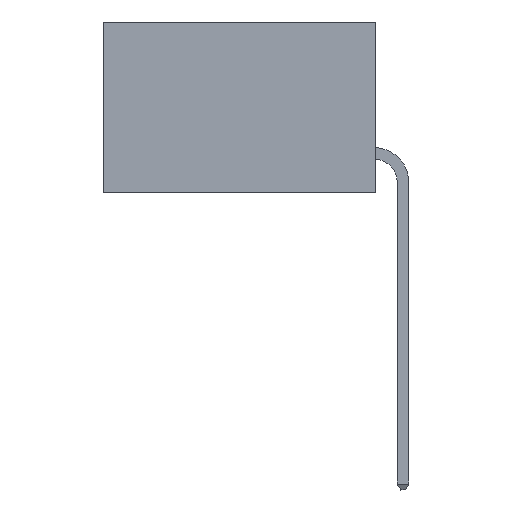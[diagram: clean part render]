
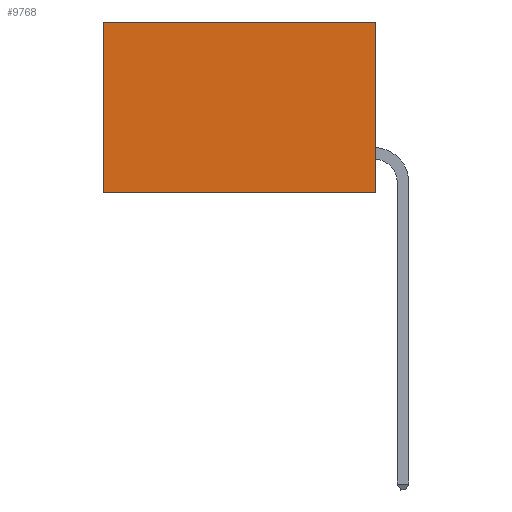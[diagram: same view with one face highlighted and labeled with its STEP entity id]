
A CAD part, left-side view. The second image highlights one B-rep face of the part: STEP entity #9768.
In plain terms, the highlighted planar face has unit normal (-1, 0, 0).
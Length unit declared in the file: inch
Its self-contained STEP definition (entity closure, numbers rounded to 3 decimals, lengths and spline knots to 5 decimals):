
#250 = EDGE_LOOP ( 'NONE', ( #1846, #6431, #14286, #9051 ) ) ;
#856 = VERTEX_POINT ( 'NONE', #9621 ) ;
#1846 = ORIENTED_EDGE ( 'NONE', *, *, #5291, .T. ) ;
#2152 = CARTESIAN_POINT ( 'NONE',  ( 0.277, 0., -0.37 ) ) ;
#2549 = CARTESIAN_POINT ( 'NONE',  ( 0.277, 0., -0.37 ) ) ;
#2844 = CARTESIAN_POINT ( 'NONE',  ( 0.277, 0., -0.37 ) ) ;
#3000 = CARTESIAN_POINT ( 'NONE',  ( 0.277, 0., -0.37 ) ) ;
#3125 = LINE ( 'NONE', #2844, #11781 ) ;
#3521 = VERTEX_POINT ( 'NONE', #2152 ) ;
#3768 = CARTESIAN_POINT ( 'NONE',  ( 0.277, 0.59, -0.37 ) ) ;
#4004 = DIRECTION ( 'NONE',  ( 0., 0., -1. ) ) ;
#4199 = CARTESIAN_POINT ( 'NONE',  ( 0.277, 0., 0. ) ) ;
#5291 = EDGE_CURVE ( 'NONE', #856, #6510, #9659, .T. ) ;
#5537 = CARTESIAN_POINT ( 'NONE',  ( 0.277, 0.59, -0.37 ) ) ;
#6286 = VECTOR ( 'NONE', #9581, 39.37008 ) ;
#6431 = ORIENTED_EDGE ( 'NONE', *, *, #11340, .F. ) ;
#6435 = CARTESIAN_POINT ( 'NONE',  ( 0.277, 0., 0. ) ) ;
#6510 = VERTEX_POINT ( 'NONE', #5537 ) ;
#7494 = FACE_OUTER_BOUND ( 'NONE', #250, .T. ) ;
#7631 = DIRECTION ( 'NONE',  ( 0., 1., 0. ) ) ;
#7711 = DIRECTION ( 'NONE',  ( 0., 0., -1. ) ) ;
#8093 = EDGE_CURVE ( 'NONE', #10435, #3521, #3125, .T. ) ;
#8206 = VECTOR ( 'NONE', #7631, 39.37008 ) ;
#8801 = AXIS2_PLACEMENT_3D ( 'NONE', #3000, #14757, #7711 ) ;
#9002 = EDGE_CURVE ( 'NONE', #10435, #856, #14499, .T. ) ;
#9051 = ORIENTED_EDGE ( 'NONE', *, *, #9002, .T. ) ;
#9581 = DIRECTION ( 'NONE',  ( 0., 1., 0. ) ) ;
#9621 = CARTESIAN_POINT ( 'NONE',  ( 0.277, 0.59, 0. ) ) ;
#9659 = LINE ( 'NONE', #3768, #12808 ) ;
#9768 = ADVANCED_FACE ( 'NONE', ( #7494 ), #12412, .F. ) ;
#9798 = LINE ( 'NONE', #2549, #6286 ) ;
#10435 = VERTEX_POINT ( 'NONE', #4199 ) ;
#11079 = DIRECTION ( 'NONE',  ( 0., 0., -1. ) ) ;
#11340 = EDGE_CURVE ( 'NONE', #3521, #6510, #9798, .T. ) ;
#11781 = VECTOR ( 'NONE', #11079, 39.37008 ) ;
#12412 = PLANE ( 'NONE',  #8801 ) ;
#12808 = VECTOR ( 'NONE', #4004, 39.37008 ) ;
#14286 = ORIENTED_EDGE ( 'NONE', *, *, #8093, .F. ) ;
#14499 = LINE ( 'NONE', #6435, #8206 ) ;
#14757 = DIRECTION ( 'NONE',  ( 1., 0., 0. ) ) ;
